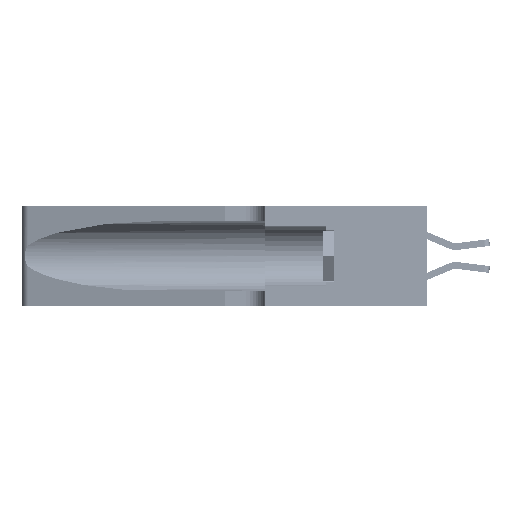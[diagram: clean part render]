
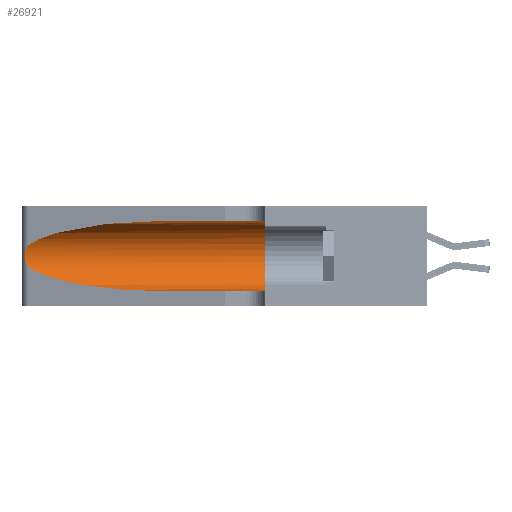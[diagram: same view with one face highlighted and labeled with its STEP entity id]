
A CAD part, left-side view. The second image highlights one B-rep face of the part: STEP entity #26921.
In plain terms, the highlighted cylindrical face has radius 3.308 mm (diameter 6.617 mm), a partial arc.
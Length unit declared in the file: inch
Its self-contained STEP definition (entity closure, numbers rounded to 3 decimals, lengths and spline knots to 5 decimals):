
#941 = CARTESIAN_POINT ( 'NONE',  ( 0.1305, 0.72297, 0.05475 ) ) ;
#1709 = CARTESIAN_POINT ( 'NONE',  ( 0.25787, 1.23484, 0.2124 ) ) ;
#2181 = ORIENTED_EDGE ( 'NONE', *, *, #28133, .F. ) ;
#2462 = LINE ( 'NONE', #28095, #32489 ) ;
#5271 = CARTESIAN_POINT ( 'NONE',  ( 0.1305, 0.72297, 0.31525 ) ) ;
#5614 = DIRECTION ( 'NONE',  ( 0., -1., 0. ) ) ;
#5790 = CARTESIAN_POINT ( 'NONE',  ( 0.26018, 1.23835, 0.19895 ) ) ;
#6503 = VECTOR ( 'NONE', #41037, 39.37008 ) ;
#7031 = CARTESIAN_POINT ( 'NONE',  ( 0.2373, 1.15595, 0.08982 ) ) ;
#7508 = ORIENTED_EDGE ( 'NONE', *, *, #10105, .T. ) ;
#8192 = CARTESIAN_POINT ( 'NONE',  ( 0.25487, 1.22718, 0.14631 ) ) ;
#8525 = DIRECTION ( 'NONE',  ( 0., -1., 0. ) ) ;
#9405 = EDGE_LOOP ( 'NONE', ( #36573, #11464, #46770, #7508, #35493, #2181 ) ) ;
#9831 = CARTESIAN_POINT ( 'NONE',  ( 0.26075, 1.23896, 0.178 ) ) ;
#10105 = EDGE_CURVE ( 'NONE', #11679, #16271, #17063, .T. ) ;
#11024 = EDGE_CURVE ( 'NONE', #35839, #34539, #34872, .T. ) ;
#11029 = CARTESIAN_POINT ( 'NONE',  ( 0.18966, 0.96281, 0.05475 ) ) ;
#11464 = ORIENTED_EDGE ( 'NONE', *, *, #44934, .T. ) ;
#11679 = VERTEX_POINT ( 'NONE', #941 ) ;
#13649 = DIRECTION ( 'NONE',  ( 0., 0., -1. ) ) ;
#13827 = CARTESIAN_POINT ( 'NONE',  ( 0.25856, 1.23593, 0.16098 ) ) ;
#16271 = VERTEX_POINT ( 'NONE', #24367 ) ;
#17024 = CARTESIAN_POINT ( 'NONE',  ( 0.1305, 0.35, 0.31525 ) ) ;
#17063 = LINE ( 'NONE', #18050, #6503 ) ;
#17772 = CARTESIAN_POINT ( 'NONE',  ( 0.25639, 1.23186, 0.15144 ) ) ;
#18050 = CARTESIAN_POINT ( 'NONE',  ( 0.1305, 1.61858, 0.05475 ) ) ;
#18350 = CARTESIAN_POINT ( 'NONE',  ( 0.1305, 0.72297, 0.31525 ) ) ;
#18907 = CARTESIAN_POINT ( 'NONE',  ( 0.1305, 0.35, 0.185 ) ) ;
#20991 = CARTESIAN_POINT ( 'NONE',  ( 0.18966, 0.96281, 0.31525 ) ) ;
#21481 = CARTESIAN_POINT ( 'NONE',  ( 0.25487, 1.22718, 0.22369 ) ) ;
#21486 = VERTEX_POINT ( 'NONE', #8192 ) ;
#21638 = CARTESIAN_POINT ( 'NONE',  ( 0.25487, 1.22718, 0.14631 ) ) ;
#22752 = DIRECTION ( 'NONE',  ( 0., 0., 1. ) ) ;
#24367 = CARTESIAN_POINT ( 'NONE',  ( 0.1305, 0.35, 0.05475 ) ) ;
#25330 = CARTESIAN_POINT ( 'NONE',  ( 0.25639, 1.23184, 0.21858 ) ) ;
#26473 = CARTESIAN_POINT ( 'NONE',  ( 0.25487, 1.22718, 0.14631 ) ) ;
#26921 = ADVANCED_FACE ( 'NONE', ( #29014 ), #48226, .F. ) ;
#28095 = CARTESIAN_POINT ( 'NONE',  ( 0.1305, 1.61858, 0.31525 ) ) ;
#28133 = EDGE_CURVE ( 'NONE', #35839, #35632, #2462, .T. ) ;
#29014 = FACE_OUTER_BOUND ( 'NONE', #9405, .T. ) ;
#29186 = CARTESIAN_POINT ( 'NONE',  ( 0.25854, 1.2359, 0.20912 ) ) ;
#29642 = CIRCLE ( 'NONE', #43077, 0.13025 ) ;
#32489 = VECTOR ( 'NONE', #8525, 39.37008 ) ;
#32562 = CARTESIAN_POINT ( 'NONE',  ( 0.25487, 1.22718, 0.22369 ) ) ;
#32710 =( BOUNDED_CURVE ( )  B_SPLINE_CURVE ( 3, ( #26473, #7031, #11029, #38049 ),
 .UNSPECIFIED., .F., .F. ) 
 B_SPLINE_CURVE_WITH_KNOTS ( ( 4, 4 ),
 ( 3.44316, 4.71239 ),
 .UNSPECIFIED. ) 
 CURVE ( )  GEOMETRIC_REPRESENTATION_ITEM ( )  RATIONAL_B_SPLINE_CURVE ( ( 1., 0.87, 0.87, 1. ) ) 
 REPRESENTATION_ITEM ( '' )  );
#33040 = CARTESIAN_POINT ( 'NONE',  ( 0.26075, 1.23896, 0.19203 ) ) ;
#34539 = VERTEX_POINT ( 'NONE', #39401 ) ;
#34872 =( BOUNDED_CURVE ( )  B_SPLINE_CURVE ( 3, ( #5271, #20991, #43922, #32562 ),
 .UNSPECIFIED., .F., .F. ) 
 B_SPLINE_CURVE_WITH_KNOTS ( ( 4, 4 ),
 ( 1.5708, 2.84003 ),
 .UNSPECIFIED. ) 
 CURVE ( )  GEOMETRIC_REPRESENTATION_ITEM ( )  RATIONAL_B_SPLINE_CURVE ( ( 1., 0.87, 0.87, 1. ) ) 
 REPRESENTATION_ITEM ( '' )  );
#35493 = ORIENTED_EDGE ( 'NONE', *, *, #37279, .F. ) ;
#35632 = VERTEX_POINT ( 'NONE', #17024 ) ;
#35839 = VERTEX_POINT ( 'NONE', #18350 ) ;
#36573 = ORIENTED_EDGE ( 'NONE', *, *, #11024, .T. ) ;
#36882 = CARTESIAN_POINT ( 'NONE',  ( 0.26017, 1.23833, 0.17102 ) ) ;
#37279 = EDGE_CURVE ( 'NONE', #35632, #16271, #29642, .T. ) ;
#38049 = CARTESIAN_POINT ( 'NONE',  ( 0.1305, 0.72297, 0.05475 ) ) ;
#39401 = CARTESIAN_POINT ( 'NONE',  ( 0.25487, 1.22718, 0.22369 ) ) ;
#40588 = CARTESIAN_POINT ( 'NONE',  ( 0.1305, 1.61858, 0.185 ) ) ;
#40750 = CARTESIAN_POINT ( 'NONE',  ( 0.25789, 1.23486, 0.15765 ) ) ;
#41037 = DIRECTION ( 'NONE',  ( 0., -1., 0. ) ) ;
#41621 = B_SPLINE_CURVE_WITH_KNOTS ( 'NONE', 3,
 ( #21481, #44421, #25330, #1709, #29186, #5790, #33040, #9831, #36882, #13827, #40750, #17772, #44594, #21638 ),
 .UNSPECIFIED., .F., .F.,
 ( 4, 2, 2, 2, 2, 2, 4 ),
 ( 0., 0.00027, 0.00053, 0.00107, 0.0016, 0.00187, 0.00214 ),
 .UNSPECIFIED. ) ;
#43077 = AXIS2_PLACEMENT_3D ( 'NONE', #18907, #45716, #22752 ) ;
#43922 = CARTESIAN_POINT ( 'NONE',  ( 0.2373, 1.15595, 0.28018 ) ) ;
#44421 = CARTESIAN_POINT ( 'NONE',  ( 0.25555, 1.22994, 0.2215 ) ) ;
#44594 = CARTESIAN_POINT ( 'NONE',  ( 0.25555, 1.22993, 0.14849 ) ) ;
#44934 = EDGE_CURVE ( 'NONE', #34539, #21486, #41621, .T. ) ;
#45134 = EDGE_CURVE ( 'NONE', #21486, #11679, #32710, .T. ) ;
#45347 = AXIS2_PLACEMENT_3D ( 'NONE', #40588, #5614, #13649 ) ;
#45716 = DIRECTION ( 'NONE',  ( 0., 1., 0. ) ) ;
#46770 = ORIENTED_EDGE ( 'NONE', *, *, #45134, .T. ) ;
#48226 = CYLINDRICAL_SURFACE ( 'NONE', #45347, 0.13025 ) ;
